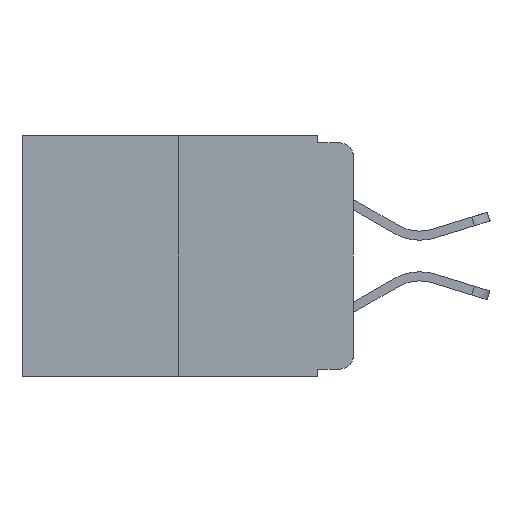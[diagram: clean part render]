
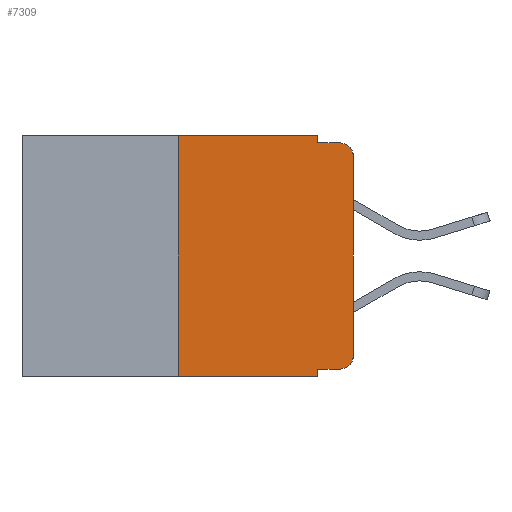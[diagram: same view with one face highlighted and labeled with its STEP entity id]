
A CAD part, left-side view. The second image highlights one B-rep face of the part: STEP entity #7309.
In plain terms, the highlighted planar face has unit normal (-1, 0, 0).
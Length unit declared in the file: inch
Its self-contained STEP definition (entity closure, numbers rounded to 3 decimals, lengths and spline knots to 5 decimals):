
#201 = VERTEX_POINT ( 'NONE', #6718 ) ;
#204 = LINE ( 'NONE', #6775, #19494 ) ;
#350 = LINE ( 'NONE', #8709, #15393 ) ;
#1623 = ORIENTED_EDGE ( 'NONE', *, *, #25264, .T. ) ;
#2023 = CARTESIAN_POINT ( 'NONE',  ( 0., 0., 0. ) ) ;
#2062 = ORIENTED_EDGE ( 'NONE', *, *, #2104, .F. ) ;
#2104 = EDGE_CURVE ( 'NONE', #201, #11060, #8427, .T. ) ;
#2289 = VERTEX_POINT ( 'NONE', #3826 ) ;
#2293 = VERTEX_POINT ( 'NONE', #13927 ) ;
#2393 = ORIENTED_EDGE ( 'NONE', *, *, #2917, .T. ) ;
#2419 = CARTESIAN_POINT ( 'NONE',  ( 0., 0., -0.03 ) ) ;
#2694 = EDGE_CURVE ( 'NONE', #20649, #201, #4632, .T. ) ;
#2792 = PLANE ( 'NONE',  #20905 ) ;
#2917 = EDGE_CURVE ( 'NONE', #7633, #11526, #24564, .T. ) ;
#3481 = CARTESIAN_POINT ( 'NONE',  ( 0., 0.051, -0.333 ) ) ;
#3612 = CARTESIAN_POINT ( 'NONE',  ( 0., 0.051, 0. ) ) ;
#3630 = ORIENTED_EDGE ( 'NONE', *, *, #12667, .T. ) ;
#3826 = CARTESIAN_POINT ( 'NONE',  ( 0., 0.02, -0.01 ) ) ;
#4035 = DIRECTION ( 'NONE',  ( 0., 0., 1. ) ) ;
#4632 = LINE ( 'NONE', #16642, #15261 ) ;
#6390 = EDGE_CURVE ( 'NONE', #12816, #7633, #20529, .T. ) ;
#6718 = CARTESIAN_POINT ( 'NONE',  ( 0., 0.25, 0. ) ) ;
#6775 = CARTESIAN_POINT ( 'NONE',  ( 0., 0.051, -0.333 ) ) ;
#7309 = ADVANCED_FACE ( 'NONE', ( #13955 ), #2792, .F. ) ;
#7384 = CARTESIAN_POINT ( 'NONE',  ( 0., 0.051, -0.343 ) ) ;
#7633 = VERTEX_POINT ( 'NONE', #17237 ) ;
#7733 = VECTOR ( 'NONE', #12821, 39.37008 ) ;
#8086 = EDGE_CURVE ( 'NONE', #11526, #2289, #12387, .T. ) ;
#8266 = DIRECTION ( 'NONE',  ( 0., 0., -1. ) ) ;
#8427 = LINE ( 'NONE', #19006, #18319 ) ;
#8585 = CARTESIAN_POINT ( 'NONE',  ( 0., 0.051, 0. ) ) ;
#8709 = CARTESIAN_POINT ( 'NONE',  ( 0., 0.051, 0. ) ) ;
#8946 = CARTESIAN_POINT ( 'NONE',  ( 0., 0.051, -0.01 ) ) ;
#9308 = ORIENTED_EDGE ( 'NONE', *, *, #15781, .F. ) ;
#9467 = DIRECTION ( 'NONE',  ( -1., 0., 0. ) ) ;
#10797 = DIRECTION ( 'NONE',  ( 0., 0., -1. ) ) ;
#10800 = CARTESIAN_POINT ( 'NONE',  ( 0., 0.473, -0.343 ) ) ;
#10909 = DIRECTION ( 'NONE',  ( 0., 0., 1. ) ) ;
#11060 = VERTEX_POINT ( 'NONE', #8585 ) ;
#11526 = VERTEX_POINT ( 'NONE', #2419 ) ;
#11739 = VECTOR ( 'NONE', #24527, 39.37008 ) ;
#12387 = CIRCLE ( 'NONE', #17382, 0.02 ) ;
#12667 = EDGE_CURVE ( 'NONE', #20649, #16498, #24565, .T. ) ;
#12816 = VERTEX_POINT ( 'NONE', #17074 ) ;
#12821 = DIRECTION ( 'NONE',  ( 0., -1., 0. ) ) ;
#13393 = ORIENTED_EDGE ( 'NONE', *, *, #2694, .F. ) ;
#13635 = DIRECTION ( 'NONE',  ( 0., 0., -1. ) ) ;
#13712 = ORIENTED_EDGE ( 'NONE', *, *, #8086, .T. ) ;
#13927 = CARTESIAN_POINT ( 'NONE',  ( 0., 0.051, -0.01 ) ) ;
#13955 = FACE_OUTER_BOUND ( 'NONE', #15452, .T. ) ;
#14759 = DIRECTION ( 'NONE',  ( 0., -1., 0. ) ) ;
#15261 = VECTOR ( 'NONE', #10909, 39.37008 ) ;
#15393 = VECTOR ( 'NONE', #20365, 39.37008 ) ;
#15452 = EDGE_LOOP ( 'NONE', ( #2393, #13712, #9308, #21538, #2062, #13393, #3630, #25136, #1623, #16941 ) ) ;
#15781 = EDGE_CURVE ( 'NONE', #2293, #2289, #16353, .T. ) ;
#16353 = LINE ( 'NONE', #8946, #11739 ) ;
#16431 = CARTESIAN_POINT ( 'NONE',  ( 0., 0.02, -0.03 ) ) ;
#16498 = VERTEX_POINT ( 'NONE', #7384 ) ;
#16565 = EDGE_CURVE ( 'NONE', #17627, #16498, #21998, .T. ) ;
#16642 = CARTESIAN_POINT ( 'NONE',  ( 0., 0.25, 0. ) ) ;
#16739 = CARTESIAN_POINT ( 'NONE',  ( 0., 0.473, 0. ) ) ;
#16917 = VECTOR ( 'NONE', #13635, 39.37008 ) ;
#16941 = ORIENTED_EDGE ( 'NONE', *, *, #6390, .T. ) ;
#17074 = CARTESIAN_POINT ( 'NONE',  ( 0., 0.02, -0.333 ) ) ;
#17237 = CARTESIAN_POINT ( 'NONE',  ( 0., 0., -0.313 ) ) ;
#17382 = AXIS2_PLACEMENT_3D ( 'NONE', #16431, #20817, #18607 ) ;
#17627 = VERTEX_POINT ( 'NONE', #3481 ) ;
#18136 = AXIS2_PLACEMENT_3D ( 'NONE', #22958, #9467, #8266 ) ;
#18319 = VECTOR ( 'NONE', #19254, 39.37008 ) ;
#18607 = DIRECTION ( 'NONE',  ( 0., 0., -1. ) ) ;
#19006 = CARTESIAN_POINT ( 'NONE',  ( 0., 0.473, 0. ) ) ;
#19254 = DIRECTION ( 'NONE',  ( 0., -1., 0. ) ) ;
#19456 = VECTOR ( 'NONE', #4035, 39.37008 ) ;
#19494 = VECTOR ( 'NONE', #14759, 39.37008 ) ;
#20323 = CARTESIAN_POINT ( 'NONE',  ( 0., 0.25, -0.343 ) ) ;
#20365 = DIRECTION ( 'NONE',  ( 0., 0., -1. ) ) ;
#20529 = CIRCLE ( 'NONE', #18136, 0.02 ) ;
#20649 = VERTEX_POINT ( 'NONE', #20323 ) ;
#20817 = DIRECTION ( 'NONE',  ( -1., 0., 0. ) ) ;
#20905 = AXIS2_PLACEMENT_3D ( 'NONE', #16739, #22420, #10797 ) ;
#21538 = ORIENTED_EDGE ( 'NONE', *, *, #23299, .F. ) ;
#21998 = LINE ( 'NONE', #3612, #16917 ) ;
#22420 = DIRECTION ( 'NONE',  ( 1., 0., 0. ) ) ;
#22958 = CARTESIAN_POINT ( 'NONE',  ( 0., 0.02, -0.313 ) ) ;
#23299 = EDGE_CURVE ( 'NONE', #11060, #2293, #350, .T. ) ;
#24527 = DIRECTION ( 'NONE',  ( 0., -1., 0. ) ) ;
#24564 = LINE ( 'NONE', #2023, #19456 ) ;
#24565 = LINE ( 'NONE', #10800, #7733 ) ;
#25136 = ORIENTED_EDGE ( 'NONE', *, *, #16565, .F. ) ;
#25264 = EDGE_CURVE ( 'NONE', #17627, #12816, #204, .T. ) ;
